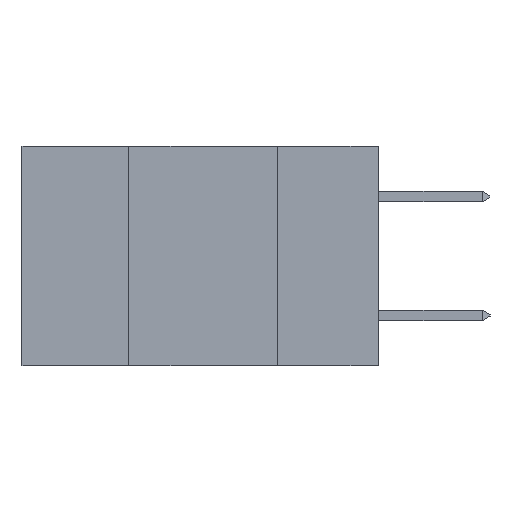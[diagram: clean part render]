
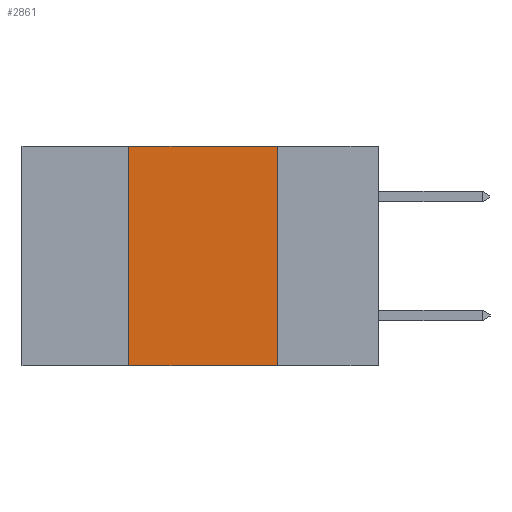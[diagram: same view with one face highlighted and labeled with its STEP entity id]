
A CAD part, left-side view. The second image highlights one B-rep face of the part: STEP entity #2861.
In plain terms, the highlighted planar face has unit normal (-1, 0, 0).
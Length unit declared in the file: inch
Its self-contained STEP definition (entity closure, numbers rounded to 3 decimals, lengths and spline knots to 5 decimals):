
#2159 = CARTESIAN_POINT ( 'NONE',  ( 0., 0.42, 0. ) ) ;
#2266 = ORIENTED_EDGE ( 'NONE', *, *, #8263, .F. ) ;
#2352 = CARTESIAN_POINT ( 'NONE',  ( 0., 0.42, -0.37 ) ) ;
#2861 = ADVANCED_FACE ( 'NONE', ( #17012 ), #9391, .F. ) ;
#3980 = CARTESIAN_POINT ( 'NONE',  ( 0., 0.6, -0.37 ) ) ;
#5073 = VERTEX_POINT ( 'NONE', #2159 ) ;
#5180 = ORIENTED_EDGE ( 'NONE', *, *, #5395, .F. ) ;
#5395 = EDGE_CURVE ( 'NONE', #5073, #6477, #13520, .T. ) ;
#5457 = DIRECTION ( 'NONE',  ( 0., -1., 0. ) ) ;
#6477 = VERTEX_POINT ( 'NONE', #15938 ) ;
#7181 = EDGE_LOOP ( 'NONE', ( #2266, #5180, #16553, #10539 ) ) ;
#7227 = DIRECTION ( 'NONE',  ( 0., 0., -1. ) ) ;
#7668 = VERTEX_POINT ( 'NONE', #17188 ) ;
#7989 = DIRECTION ( 'NONE',  ( 1., 0., 0. ) ) ;
#8263 = EDGE_CURVE ( 'NONE', #6477, #7668, #12708, .T. ) ;
#8618 = LINE ( 'NONE', #3980, #15580 ) ;
#8641 = CARTESIAN_POINT ( 'NONE',  ( 0., 0.6, 0. ) ) ;
#9391 = PLANE ( 'NONE',  #16252 ) ;
#9925 = VERTEX_POINT ( 'NONE', #12916 ) ;
#10539 = ORIENTED_EDGE ( 'NONE', *, *, #14797, .T. ) ;
#10718 = VECTOR ( 'NONE', #5457, 39.37008 ) ;
#12708 = LINE ( 'NONE', #17836, #15930 ) ;
#12916 = CARTESIAN_POINT ( 'NONE',  ( 0., 0.42, -0.37 ) ) ;
#13520 = LINE ( 'NONE', #13862, #10718 ) ;
#13761 = LINE ( 'NONE', #2352, #16965 ) ;
#13798 = DIRECTION ( 'NONE',  ( 0., 0., -1. ) ) ;
#13862 = CARTESIAN_POINT ( 'NONE',  ( 0., 0.6, 0. ) ) ;
#14797 = EDGE_CURVE ( 'NONE', #9925, #7668, #8618, .T. ) ;
#15192 = DIRECTION ( 'NONE',  ( 0., -1., 0. ) ) ;
#15580 = VECTOR ( 'NONE', #15192, 39.37008 ) ;
#15930 = VECTOR ( 'NONE', #13798, 39.37008 ) ;
#15938 = CARTESIAN_POINT ( 'NONE',  ( 0., 0.17, 0. ) ) ;
#16252 = AXIS2_PLACEMENT_3D ( 'NONE', #8641, #7989, #7227 ) ;
#16329 = DIRECTION ( 'NONE',  ( 0., 0., 1. ) ) ;
#16553 = ORIENTED_EDGE ( 'NONE', *, *, #16612, .F. ) ;
#16612 = EDGE_CURVE ( 'NONE', #9925, #5073, #13761, .T. ) ;
#16965 = VECTOR ( 'NONE', #16329, 39.37008 ) ;
#17012 = FACE_OUTER_BOUND ( 'NONE', #7181, .T. ) ;
#17188 = CARTESIAN_POINT ( 'NONE',  ( 0., 0.17, -0.37 ) ) ;
#17836 = CARTESIAN_POINT ( 'NONE',  ( 0., 0.17, -0.37 ) ) ;
